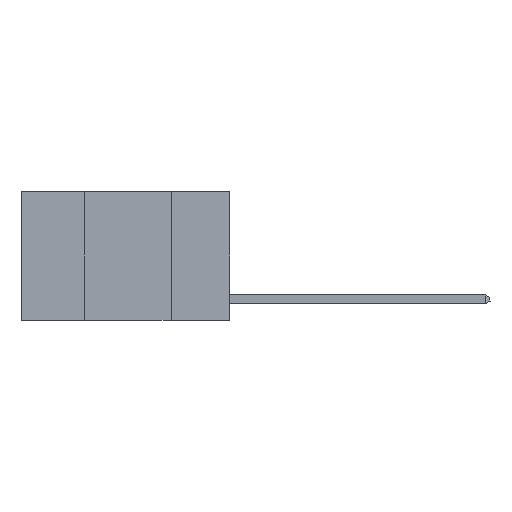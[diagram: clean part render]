
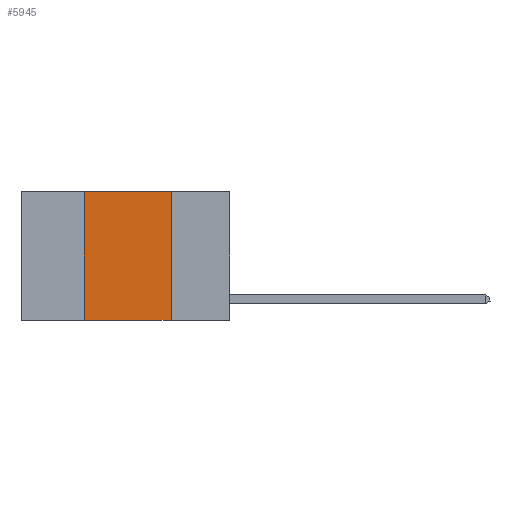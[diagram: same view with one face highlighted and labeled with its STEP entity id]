
A CAD part, left-side view. The second image highlights one B-rep face of the part: STEP entity #5945.
In plain terms, the highlighted planar face has unit normal (-1, 0, 0).
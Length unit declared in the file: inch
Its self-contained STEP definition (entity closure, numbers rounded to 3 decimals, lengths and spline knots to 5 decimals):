
#1558 = VERTEX_POINT ( 'NONE', #27483 ) ;
#1738 = DIRECTION ( 'NONE',  ( 0., -1., 0. ) ) ;
#3097 = VERTEX_POINT ( 'NONE', #4267 ) ;
#4194 = ORIENTED_EDGE ( 'NONE', *, *, #15166, .T. ) ;
#4267 = CARTESIAN_POINT ( 'NONE',  ( 0., 0.17, 0. ) ) ;
#4714 = VECTOR ( 'NONE', #5191, 39.37008 ) ;
#5163 = EDGE_LOOP ( 'NONE', ( #9809, #8405, #10809, #4194 ) ) ;
#5191 = DIRECTION ( 'NONE',  ( 0., 0., 1. ) ) ;
#5945 = ADVANCED_FACE ( 'NONE', ( #10779 ), #22479, .F. ) ;
#8405 = ORIENTED_EDGE ( 'NONE', *, *, #21626, .F. ) ;
#8506 = LINE ( 'NONE', #19004, #21121 ) ;
#9211 = EDGE_CURVE ( 'NONE', #3097, #1558, #8506, .T. ) ;
#9769 = AXIS2_PLACEMENT_3D ( 'NONE', #22390, #26931, #13538 ) ;
#9809 = ORIENTED_EDGE ( 'NONE', *, *, #9211, .F. ) ;
#10779 = FACE_OUTER_BOUND ( 'NONE', #5163, .T. ) ;
#10809 = ORIENTED_EDGE ( 'NONE', *, *, #13652, .F. ) ;
#12275 = VECTOR ( 'NONE', #1738, 39.37008 ) ;
#13538 = DIRECTION ( 'NONE',  ( 0., 0., -1. ) ) ;
#13652 = EDGE_CURVE ( 'NONE', #15091, #17909, #16579, .T. ) ;
#15091 = VERTEX_POINT ( 'NONE', #19305 ) ;
#15166 = EDGE_CURVE ( 'NONE', #15091, #1558, #17552, .T. ) ;
#16579 = LINE ( 'NONE', #18597, #4714 ) ;
#17333 = CARTESIAN_POINT ( 'NONE',  ( 0., 0.6, -0.37 ) ) ;
#17552 = LINE ( 'NONE', #17333, #12275 ) ;
#17909 = VERTEX_POINT ( 'NONE', #27784 ) ;
#18298 = VECTOR ( 'NONE', #27744, 39.37008 ) ;
#18597 = CARTESIAN_POINT ( 'NONE',  ( 0., 0.42, 0. ) ) ;
#18910 = DIRECTION ( 'NONE',  ( 0., 0., -1. ) ) ;
#19004 = CARTESIAN_POINT ( 'NONE',  ( 0., 0.17, 0. ) ) ;
#19305 = CARTESIAN_POINT ( 'NONE',  ( 0., 0.42, -0.37 ) ) ;
#21065 = CARTESIAN_POINT ( 'NONE',  ( 0., 0.6, 0. ) ) ;
#21121 = VECTOR ( 'NONE', #18910, 39.37008 ) ;
#21626 = EDGE_CURVE ( 'NONE', #17909, #3097, #24923, .T. ) ;
#22390 = CARTESIAN_POINT ( 'NONE',  ( 0., 0.6, 0. ) ) ;
#22479 = PLANE ( 'NONE',  #9769 ) ;
#24923 = LINE ( 'NONE', #21065, #18298 ) ;
#26931 = DIRECTION ( 'NONE',  ( 1., 0., 0. ) ) ;
#27483 = CARTESIAN_POINT ( 'NONE',  ( 0., 0.17, -0.37 ) ) ;
#27744 = DIRECTION ( 'NONE',  ( 0., -1., 0. ) ) ;
#27784 = CARTESIAN_POINT ( 'NONE',  ( 0., 0.42, 0. ) ) ;
